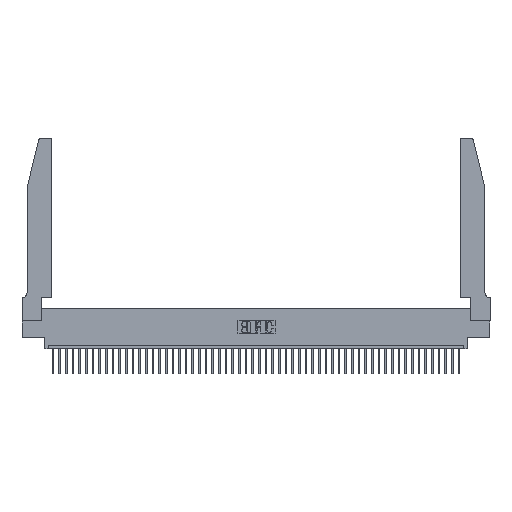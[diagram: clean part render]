
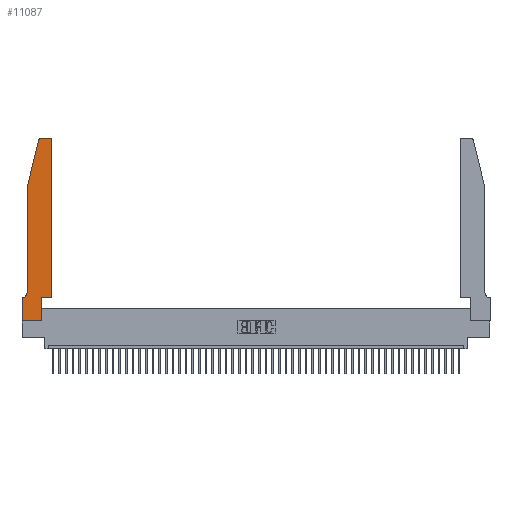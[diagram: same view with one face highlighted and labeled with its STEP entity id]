
A CAD part, top view. The second image highlights one B-rep face of the part: STEP entity #11087.
In plain terms, the highlighted planar face has unit normal (0, 0, 1).
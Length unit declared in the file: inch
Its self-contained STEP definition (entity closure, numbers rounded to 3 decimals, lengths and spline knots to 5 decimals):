
#646 = ORIENTED_EDGE ( 'NONE', *, *, #42251, .T. ) ;
#1116 = FACE_OUTER_BOUND ( 'NONE', #48745, .T. ) ;
#1572 = CIRCLE ( 'NONE', #7722, 0.03 ) ;
#1595 = CARTESIAN_POINT ( 'NONE',  ( 0.4205, 2.75, 0.37 ) ) ;
#2186 = VERTEX_POINT ( 'NONE', #48217 ) ;
#2278 = CARTESIAN_POINT ( 'NONE',  ( 0.0755, 0.42, 0.37 ) ) ;
#3010 = ORIENTED_EDGE ( 'NONE', *, *, #35734, .T. ) ;
#4010 = VERTEX_POINT ( 'NONE', #18330 ) ;
#4322 = CIRCLE ( 'NONE', #21134, 0.07 ) ;
#5003 = DIRECTION ( 'NONE',  ( 1., 0., 0. ) ) ;
#6909 = ORIENTED_EDGE ( 'NONE', *, *, #20456, .T. ) ;
#7649 = DIRECTION ( 'NONE',  ( -1., 0., 0. ) ) ;
#7713 = DIRECTION ( 'NONE',  ( 0., 1., 0. ) ) ;
#7722 = AXIS2_PLACEMENT_3D ( 'NONE', #10308, #32741, #17707 ) ;
#8934 = DIRECTION ( 'NONE',  ( -1., 0., 0. ) ) ;
#9053 = AXIS2_PLACEMENT_3D ( 'NONE', #16141, #42563, #5003 ) ;
#9484 = LINE ( 'NONE', #41533, #25356 ) ;
#9543 = CARTESIAN_POINT ( 'NONE',  ( 0., 0., 0.37 ) ) ;
#9574 = EDGE_CURVE ( 'NONE', #21812, #41537, #29029, .T. ) ;
#10308 = CARTESIAN_POINT ( 'NONE',  ( 0.4205, 2.72, 0.37 ) ) ;
#11087 = ADVANCED_FACE ( 'NONE', ( #1116 ), #21176, .T. ) ;
#11212 = ORIENTED_EDGE ( 'NONE', *, *, #19899, .T. ) ;
#11287 = LINE ( 'NONE', #46945, #18383 ) ;
#12000 = VECTOR ( 'NONE', #16423, 39.37008 ) ;
#13404 = DIRECTION ( 'NONE',  ( 0., 0., 1. ) ) ;
#13879 = DIRECTION ( 'NONE',  ( 0., 1., 0. ) ) ;
#14433 = CARTESIAN_POINT ( 'NONE',  ( 0.4505, 0.35, 0.37 ) ) ;
#15805 = CARTESIAN_POINT ( 'NONE',  ( 0.2605, 2.75, 0.37 ) ) ;
#15918 = CARTESIAN_POINT ( 'NONE',  ( 0.2865, 0., 0.37 ) ) ;
#16141 = CARTESIAN_POINT ( 'NONE',  ( 0.284, 2.72, 0.37 ) ) ;
#16423 = DIRECTION ( 'NONE',  ( 0., -1., 0. ) ) ;
#16506 = ORIENTED_EDGE ( 'NONE', *, *, #47392, .T. ) ;
#16842 = EDGE_CURVE ( 'NONE', #41440, #23092, #1572, .T. ) ;
#17080 = CARTESIAN_POINT ( 'NONE',  ( 0., 0., 0.37 ) ) ;
#17197 = CARTESIAN_POINT ( 'NONE',  ( 0., 0.35, 0.37 ) ) ;
#17240 = ORIENTED_EDGE ( 'NONE', *, *, #16842, .T. ) ;
#17564 = EDGE_CURVE ( 'NONE', #31021, #21812, #25645, .T. ) ;
#17707 = DIRECTION ( 'NONE',  ( 1., 0., 0. ) ) ;
#18330 = CARTESIAN_POINT ( 'NONE',  ( 0., 0.35, 0.37 ) ) ;
#18383 = VECTOR ( 'NONE', #47274, 39.37008 ) ;
#19479 = CARTESIAN_POINT ( 'NONE',  ( 0.2865, 0.35, 0.37 ) ) ;
#19899 = EDGE_CURVE ( 'NONE', #32125, #33620, #9484, .T. ) ;
#20456 = EDGE_CURVE ( 'NONE', #2186, #34517, #44274, .T. ) ;
#21057 = VECTOR ( 'NONE', #44635, 39.37008 ) ;
#21134 = AXIS2_PLACEMENT_3D ( 'NONE', #31475, #27682, #8934 ) ;
#21176 = PLANE ( 'NONE',  #21830 ) ;
#21526 = ORIENTED_EDGE ( 'NONE', *, *, #17564, .T. ) ;
#21812 = VERTEX_POINT ( 'NONE', #15918 ) ;
#21830 = AXIS2_PLACEMENT_3D ( 'NONE', #17197, #13404, #32202 ) ;
#23092 = VERTEX_POINT ( 'NONE', #1595 ) ;
#23226 = CARTESIAN_POINT ( 'NONE',  ( 0.0755, 0.35, 0.37 ) ) ;
#23573 = DIRECTION ( 'NONE',  ( -1., 0., 0. ) ) ;
#23912 = EDGE_CURVE ( 'NONE', #4010, #31021, #46889, .T. ) ;
#25310 = CARTESIAN_POINT ( 'NONE',  ( 0.0055, 0.35, 0.37 ) ) ;
#25348 = EDGE_CURVE ( 'NONE', #34517, #32125, #11287, .T. ) ;
#25356 = VECTOR ( 'NONE', #37447, 39.37008 ) ;
#25645 = LINE ( 'NONE', #17080, #32123 ) ;
#26141 = VERTEX_POINT ( 'NONE', #25310 ) ;
#27078 = ORIENTED_EDGE ( 'NONE', *, *, #46239, .T. ) ;
#27420 = LINE ( 'NONE', #36506, #46968 ) ;
#27516 = VECTOR ( 'NONE', #23573, 39.37008 ) ;
#27682 = DIRECTION ( 'NONE',  ( 0., 0., -1. ) ) ;
#28949 = ORIENTED_EDGE ( 'NONE', *, *, #34117, .T. ) ;
#29029 = LINE ( 'NONE', #19479, #33800 ) ;
#29933 = LINE ( 'NONE', #15805, #27516 ) ;
#30145 = CARTESIAN_POINT ( 'NONE',  ( 0.25487, 2.72718, 0.37 ) ) ;
#31021 = VERTEX_POINT ( 'NONE', #40337 ) ;
#31317 = ORIENTED_EDGE ( 'NONE', *, *, #25348, .T. ) ;
#31475 = CARTESIAN_POINT ( 'NONE',  ( 0.0055, 0.42, 0.37 ) ) ;
#32123 = VECTOR ( 'NONE', #32266, 39.37008 ) ;
#32125 = VERTEX_POINT ( 'NONE', #37896 ) ;
#32202 = DIRECTION ( 'NONE',  ( 1., 0., 0. ) ) ;
#32266 = DIRECTION ( 'NONE',  ( 1., 0., 0. ) ) ;
#32741 = DIRECTION ( 'NONE',  ( 0., 0., 1. ) ) ;
#33620 = VERTEX_POINT ( 'NONE', #2278 ) ;
#33800 = VECTOR ( 'NONE', #7713, 39.37008 ) ;
#34117 = EDGE_CURVE ( 'NONE', #33620, #26141, #4322, .T. ) ;
#34314 = ORIENTED_EDGE ( 'NONE', *, *, #23912, .T. ) ;
#34517 = VERTEX_POINT ( 'NONE', #30145 ) ;
#35295 = VECTOR ( 'NONE', #7649, 39.37008 ) ;
#35734 = EDGE_CURVE ( 'NONE', #23092, #2186, #29933, .T. ) ;
#36506 = CARTESIAN_POINT ( 'NONE',  ( 0.4505, 0.35, 0.37 ) ) ;
#37111 = CARTESIAN_POINT ( 'NONE',  ( 0.4505, 0.35, 0.37 ) ) ;
#37447 = DIRECTION ( 'NONE',  ( 0., -1., 0. ) ) ;
#37543 = CARTESIAN_POINT ( 'NONE',  ( 0.2865, 0.35, 0.37 ) ) ;
#37845 = CARTESIAN_POINT ( 'NONE',  ( 0.4505, 2.72, 0.37 ) ) ;
#37896 = CARTESIAN_POINT ( 'NONE',  ( 0.0755, 2., 0.37 ) ) ;
#38964 = VERTEX_POINT ( 'NONE', #37111 ) ;
#40337 = CARTESIAN_POINT ( 'NONE',  ( 0., 0., 0.37 ) ) ;
#41440 = VERTEX_POINT ( 'NONE', #37845 ) ;
#41533 = CARTESIAN_POINT ( 'NONE',  ( 0.0755, 2., 0.37 ) ) ;
#41537 = VERTEX_POINT ( 'NONE', #37543 ) ;
#41712 = LINE ( 'NONE', #14433, #21057 ) ;
#42251 = EDGE_CURVE ( 'NONE', #38964, #41440, #27420, .T. ) ;
#42563 = DIRECTION ( 'NONE',  ( 0., 0., 1. ) ) ;
#43607 = LINE ( 'NONE', #23226, #35295 ) ;
#43958 = ORIENTED_EDGE ( 'NONE', *, *, #9574, .T. ) ;
#44274 = CIRCLE ( 'NONE', #9053, 0.03 ) ;
#44635 = DIRECTION ( 'NONE',  ( 1., 0., 0. ) ) ;
#46239 = EDGE_CURVE ( 'NONE', #26141, #4010, #43607, .T. ) ;
#46889 = LINE ( 'NONE', #9543, #12000 ) ;
#46945 = CARTESIAN_POINT ( 'NONE',  ( 0.0755, 2., 0.37 ) ) ;
#46968 = VECTOR ( 'NONE', #13879, 39.37008 ) ;
#47274 = DIRECTION ( 'NONE',  ( -0.239, -0.971, 0. ) ) ;
#47392 = EDGE_CURVE ( 'NONE', #41537, #38964, #41712, .T. ) ;
#48217 = CARTESIAN_POINT ( 'NONE',  ( 0.284, 2.75, 0.37 ) ) ;
#48745 = EDGE_LOOP ( 'NONE', ( #3010, #6909, #31317, #11212, #28949, #27078, #34314, #21526, #43958, #16506, #646, #17240 ) ) ;
